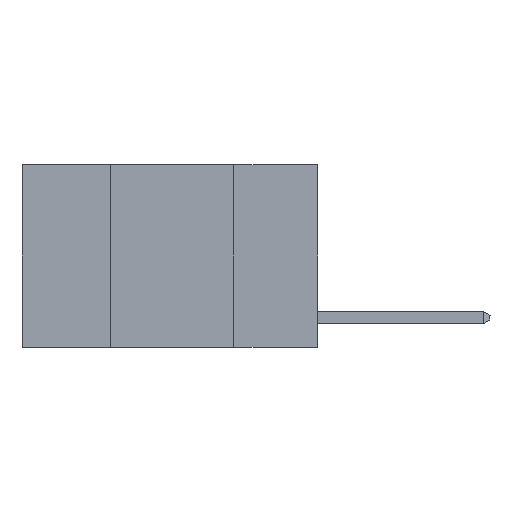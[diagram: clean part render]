
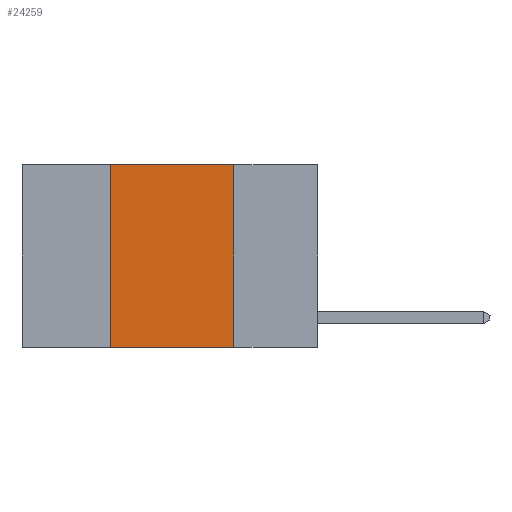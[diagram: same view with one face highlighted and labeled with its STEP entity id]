
A CAD part, left-side view. The second image highlights one B-rep face of the part: STEP entity #24259.
In plain terms, the highlighted planar face has unit normal (-1, 0, 0).
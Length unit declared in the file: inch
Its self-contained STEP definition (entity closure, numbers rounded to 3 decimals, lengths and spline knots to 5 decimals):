
#820 = EDGE_CURVE ( 'NONE', #8290, #7056, #17376, .T. ) ;
#2292 = ORIENTED_EDGE ( 'NONE', *, *, #23750, .T. ) ;
#2611 = VERTEX_POINT ( 'NONE', #8219 ) ;
#4390 = CARTESIAN_POINT ( 'NONE',  ( 0., 0.42, 0. ) ) ;
#4475 = LINE ( 'NONE', #24121, #9860 ) ;
#5661 = CARTESIAN_POINT ( 'NONE',  ( 0., 0.42, -0.37 ) ) ;
#6123 = DIRECTION ( 'NONE',  ( 0., -1., 0. ) ) ;
#6357 = VERTEX_POINT ( 'NONE', #6538 ) ;
#6376 = DIRECTION ( 'NONE',  ( 0., 0., -1. ) ) ;
#6538 = CARTESIAN_POINT ( 'NONE',  ( 0., 0.17, 0. ) ) ;
#7033 = VECTOR ( 'NONE', #6376, 39.37008 ) ;
#7056 = VERTEX_POINT ( 'NONE', #4390 ) ;
#7074 = DIRECTION ( 'NONE',  ( 1., 0., 0. ) ) ;
#7146 = EDGE_LOOP ( 'NONE', ( #12446, #23142, #12106, #2292 ) ) ;
#8219 = CARTESIAN_POINT ( 'NONE',  ( 0., 0.17, -0.37 ) ) ;
#8290 = VERTEX_POINT ( 'NONE', #5661 ) ;
#8392 = CARTESIAN_POINT ( 'NONE',  ( 0., 0.42, 0. ) ) ;
#8846 = DIRECTION ( 'NONE',  ( 0., 0., 1. ) ) ;
#9860 = VECTOR ( 'NONE', #13097, 39.37008 ) ;
#10349 = EDGE_CURVE ( 'NONE', #6357, #2611, #13708, .T. ) ;
#11504 = VECTOR ( 'NONE', #8846, 39.37008 ) ;
#12106 = ORIENTED_EDGE ( 'NONE', *, *, #820, .F. ) ;
#12446 = ORIENTED_EDGE ( 'NONE', *, *, #10349, .F. ) ;
#13097 = DIRECTION ( 'NONE',  ( 0., -1., 0. ) ) ;
#13708 = LINE ( 'NONE', #26329, #7033 ) ;
#14277 = LINE ( 'NONE', #19497, #26060 ) ;
#17376 = LINE ( 'NONE', #8392, #11504 ) ;
#18168 = PLANE ( 'NONE',  #25655 ) ;
#19497 = CARTESIAN_POINT ( 'NONE',  ( 0., 0.6, -0.37 ) ) ;
#20398 = CARTESIAN_POINT ( 'NONE',  ( 0., 0.6, 0. ) ) ;
#22603 = DIRECTION ( 'NONE',  ( 0., 0., -1. ) ) ;
#23142 = ORIENTED_EDGE ( 'NONE', *, *, #28334, .F. ) ;
#23750 = EDGE_CURVE ( 'NONE', #8290, #2611, #14277, .T. ) ;
#24121 = CARTESIAN_POINT ( 'NONE',  ( 0., 0.6, 0. ) ) ;
#24197 = FACE_OUTER_BOUND ( 'NONE', #7146, .T. ) ;
#24259 = ADVANCED_FACE ( 'NONE', ( #24197 ), #18168, .F. ) ;
#25655 = AXIS2_PLACEMENT_3D ( 'NONE', #20398, #7074, #22603 ) ;
#26060 = VECTOR ( 'NONE', #6123, 39.37008 ) ;
#26329 = CARTESIAN_POINT ( 'NONE',  ( 0., 0.17, 0. ) ) ;
#28334 = EDGE_CURVE ( 'NONE', #7056, #6357, #4475, .T. ) ;
